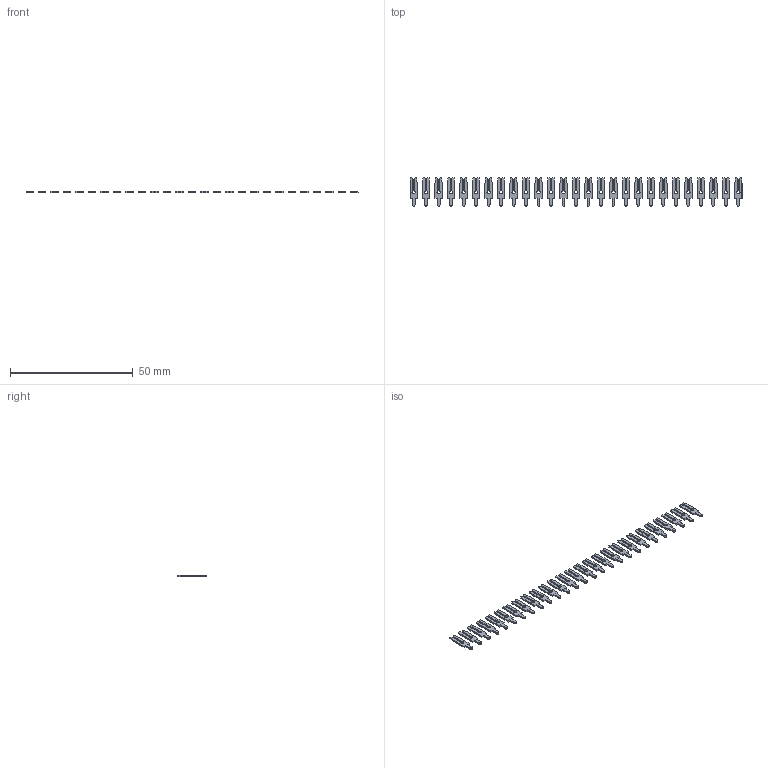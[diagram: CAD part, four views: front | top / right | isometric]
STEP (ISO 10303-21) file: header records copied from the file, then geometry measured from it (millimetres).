
FILE_DESCRIPTION (( 'STEP AP203' ), '1' );
FILE_NAME ('103-027-250-200.STEP', '2020-04-09T20:45:36', ( '' ), ( '' ), 'SwSTEP 2.0', 'SolidWorks 2016', '' );
FILE_SCHEMA (( 'CONFIG_CONTROL_DESIGN' ));
Length unit declared in the file: inch
Products named in the file (2): 100-290-001_100-290-250; 103-027-250-200
Assembly tree (27 placements, depth 2):
  103-027-250-200
    100-290-001_100-290-250  x27
Bounding box: 135 x 11.48 x 0.66 mm (x, y, z)
Volume: 421.3 mm3; surface area: 1980.4 mm2
Topology: 27 solids, 27 shells, 648 faces, 1782 edges, 1188 vertices
Faces by surface type: plane 540, cylinder 108
Entity records: 1790 total; most frequent: DIRECTION 178, CARTESIAN_POINT 176, ORIENTED_EDGE 132, EDGE_CURVE 66, COORDINATED_UNIVERSAL_TIME_OFFSET 64, CALENDAR_DATE 64, LOCAL_TIME 64, DATE_AND_TIME 64
